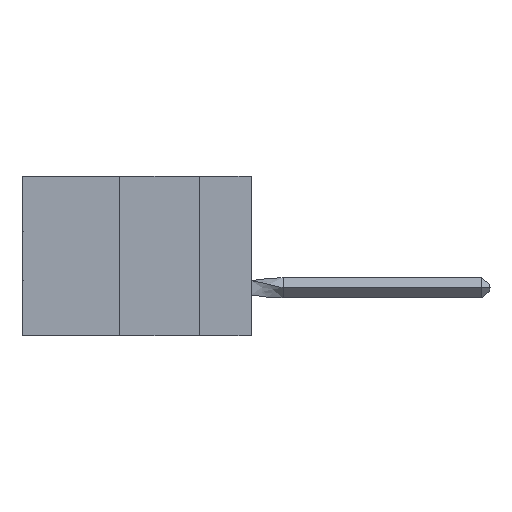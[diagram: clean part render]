
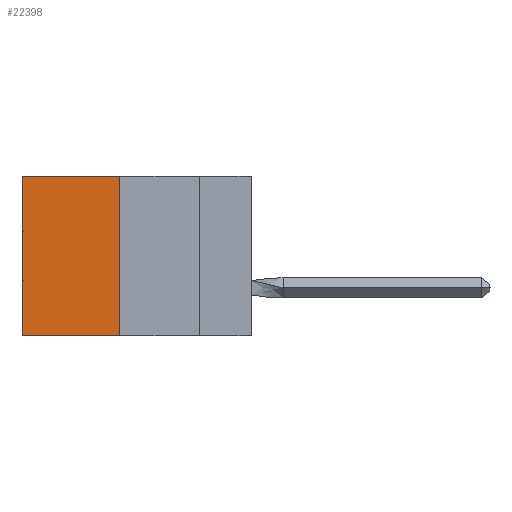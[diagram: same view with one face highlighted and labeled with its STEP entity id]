
A CAD part, left-side view. The second image highlights one B-rep face of the part: STEP entity #22398.
In plain terms, the highlighted planar face has unit normal (-1, 0, 0).
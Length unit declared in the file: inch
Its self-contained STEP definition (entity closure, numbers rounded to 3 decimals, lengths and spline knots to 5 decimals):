
#877 = ORIENTED_EDGE ( 'NONE', *, *, #34975, .T. ) ;
#879 = VECTOR ( 'NONE', #45067, 39.37008 ) ;
#2177 = DIRECTION ( 'NONE',  ( 0., 1., 0. ) ) ;
#4237 = VECTOR ( 'NONE', #29430, 39.37008 ) ;
#4337 = VERTEX_POINT ( 'NONE', #20621 ) ;
#4591 = DIRECTION ( 'NONE',  ( 0., 0., -1. ) ) ;
#4834 = VERTEX_POINT ( 'NONE', #11952 ) ;
#5759 = PLANE ( 'NONE',  #44934 ) ;
#6557 = LINE ( 'NONE', #47511, #4237 ) ;
#11376 = VERTEX_POINT ( 'NONE', #38066 ) ;
#11952 = CARTESIAN_POINT ( 'NONE',  ( 0.305, 0.413, -0.5 ) ) ;
#14234 = LINE ( 'NONE', #26221, #879 ) ;
#15737 = LINE ( 'NONE', #30622, #33737 ) ;
#16113 = EDGE_LOOP ( 'NONE', ( #877, #48023, #43322, #23815 ) ) ;
#20621 = CARTESIAN_POINT ( 'NONE',  ( 0.305, 0.72, 0. ) ) ;
#21636 = FACE_OUTER_BOUND ( 'NONE', #16113, .T. ) ;
#22398 = ADVANCED_FACE ( 'NONE', ( #21636 ), #5759, .F. ) ;
#23815 = ORIENTED_EDGE ( 'NONE', *, *, #44963, .T. ) ;
#26084 = VERTEX_POINT ( 'NONE', #34964 ) ;
#26221 = CARTESIAN_POINT ( 'NONE',  ( 0.305, 0.413, 0. ) ) ;
#29430 = DIRECTION ( 'NONE',  ( 0., 0., -1. ) ) ;
#30622 = CARTESIAN_POINT ( 'NONE',  ( 0.305, 0.413, -0.5 ) ) ;
#31299 = CARTESIAN_POINT ( 'NONE',  ( 0.305, 0.413, -0.5 ) ) ;
#33737 = VECTOR ( 'NONE', #4591, 39.37008 ) ;
#34964 = CARTESIAN_POINT ( 'NONE',  ( 0.305, 0.72, -0.5 ) ) ;
#34975 = EDGE_CURVE ( 'NONE', #4337, #26084, #6557, .T. ) ;
#35413 = EDGE_CURVE ( 'NONE', #11376, #4834, #15737, .T. ) ;
#35515 = VECTOR ( 'NONE', #2177, 39.37008 ) ;
#37265 = LINE ( 'NONE', #31299, #35515 ) ;
#38066 = CARTESIAN_POINT ( 'NONE',  ( 0.305, 0.413, 0. ) ) ;
#39160 = EDGE_CURVE ( 'NONE', #4834, #26084, #37265, .T. ) ;
#39942 = CARTESIAN_POINT ( 'NONE',  ( 0.305, 0.413, -0.5 ) ) ;
#40101 = DIRECTION ( 'NONE',  ( 0., 0., -1. ) ) ;
#43322 = ORIENTED_EDGE ( 'NONE', *, *, #35413, .F. ) ;
#44018 = DIRECTION ( 'NONE',  ( 1., 0., 0. ) ) ;
#44934 = AXIS2_PLACEMENT_3D ( 'NONE', #39942, #44018, #40101 ) ;
#44963 = EDGE_CURVE ( 'NONE', #11376, #4337, #14234, .T. ) ;
#45067 = DIRECTION ( 'NONE',  ( 0., 1., 0. ) ) ;
#47511 = CARTESIAN_POINT ( 'NONE',  ( 0.305, 0.72, -0.5 ) ) ;
#48023 = ORIENTED_EDGE ( 'NONE', *, *, #39160, .F. ) ;
